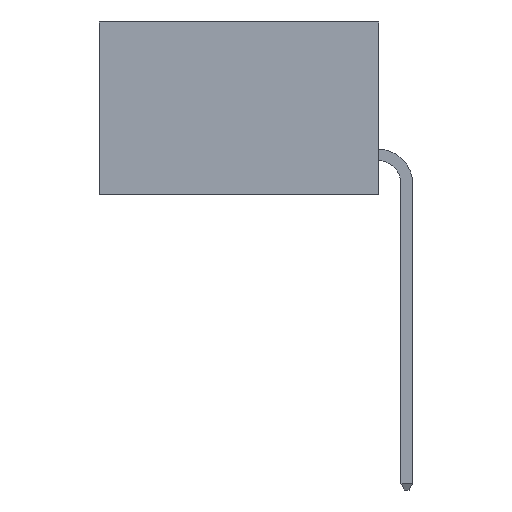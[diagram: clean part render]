
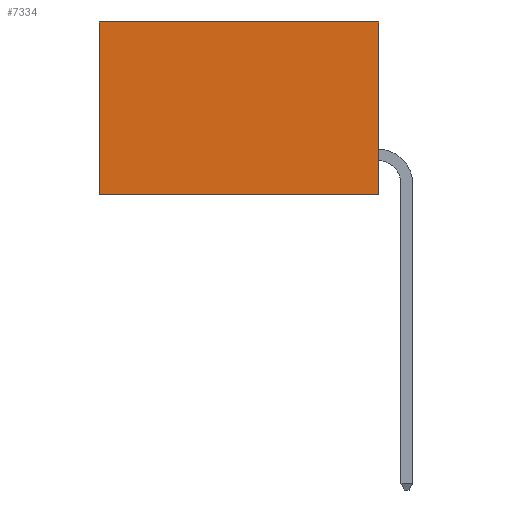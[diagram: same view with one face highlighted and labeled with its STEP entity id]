
A CAD part, left-side view. The second image highlights one B-rep face of the part: STEP entity #7334.
In plain terms, the highlighted planar face has unit normal (-1, 0, 0).
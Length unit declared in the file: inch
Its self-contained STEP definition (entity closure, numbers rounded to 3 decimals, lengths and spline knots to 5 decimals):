
#51 = VERTEX_POINT ( 'NONE', #3566 ) ;
#408 = DIRECTION ( 'NONE',  ( 0., 0., -1. ) ) ;
#463 = DIRECTION ( 'NONE',  ( 1., 0., 0. ) ) ;
#768 = VECTOR ( 'NONE', #408, 39.37008 ) ;
#1262 = EDGE_LOOP ( 'NONE', ( #2097, #7772, #4387, #2107 ) ) ;
#1339 = VERTEX_POINT ( 'NONE', #5047 ) ;
#1674 = AXIS2_PLACEMENT_3D ( 'NONE', #6868, #463, #4995 ) ;
#1951 = VECTOR ( 'NONE', #5625, 39.37008 ) ;
#2097 = ORIENTED_EDGE ( 'NONE', *, *, #4354, .T. ) ;
#2107 = ORIENTED_EDGE ( 'NONE', *, *, #7352, .T. ) ;
#2813 = DIRECTION ( 'NONE',  ( 0., 0., -1. ) ) ;
#2867 = LINE ( 'NONE', #5968, #4383 ) ;
#3528 = LINE ( 'NONE', #7677, #8002 ) ;
#3566 = CARTESIAN_POINT ( 'NONE',  ( 0.2615, 0., -0.37 ) ) ;
#3936 = FACE_OUTER_BOUND ( 'NONE', #1262, .T. ) ;
#4128 = LINE ( 'NONE', #6894, #1951 ) ;
#4274 = LINE ( 'NONE', #5570, #768 ) ;
#4354 = EDGE_CURVE ( 'NONE', #1339, #5813, #2867, .T. ) ;
#4383 = VECTOR ( 'NONE', #2813, 39.37008 ) ;
#4387 = ORIENTED_EDGE ( 'NONE', *, *, #4606, .F. ) ;
#4606 = EDGE_CURVE ( 'NONE', #5033, #51, #4274, .T. ) ;
#4995 = DIRECTION ( 'NONE',  ( 0., 0., -1. ) ) ;
#5010 = CARTESIAN_POINT ( 'NONE',  ( 0.2615, 0.6, -0.37 ) ) ;
#5033 = VERTEX_POINT ( 'NONE', #5504 ) ;
#5047 = CARTESIAN_POINT ( 'NONE',  ( 0.2615, 0.6, 0. ) ) ;
#5504 = CARTESIAN_POINT ( 'NONE',  ( 0.2615, 0., 0. ) ) ;
#5570 = CARTESIAN_POINT ( 'NONE',  ( 0.2615, 0., -0.37 ) ) ;
#5625 = DIRECTION ( 'NONE',  ( 0., 1., 0. ) ) ;
#5813 = VERTEX_POINT ( 'NONE', #5010 ) ;
#5968 = CARTESIAN_POINT ( 'NONE',  ( 0.2615, 0.6, -0.37 ) ) ;
#6868 = CARTESIAN_POINT ( 'NONE',  ( 0.2615, 0., -0.37 ) ) ;
#6894 = CARTESIAN_POINT ( 'NONE',  ( 0.2615, 0., 0. ) ) ;
#7139 = DIRECTION ( 'NONE',  ( 0., 1., 0. ) ) ;
#7334 = ADVANCED_FACE ( 'NONE', ( #3936 ), #7980, .F. ) ;
#7352 = EDGE_CURVE ( 'NONE', #5033, #1339, #4128, .T. ) ;
#7677 = CARTESIAN_POINT ( 'NONE',  ( 0.2615, 0., -0.37 ) ) ;
#7772 = ORIENTED_EDGE ( 'NONE', *, *, #8069, .F. ) ;
#7980 = PLANE ( 'NONE',  #1674 ) ;
#8002 = VECTOR ( 'NONE', #7139, 39.37008 ) ;
#8069 = EDGE_CURVE ( 'NONE', #51, #5813, #3528, .T. ) ;
